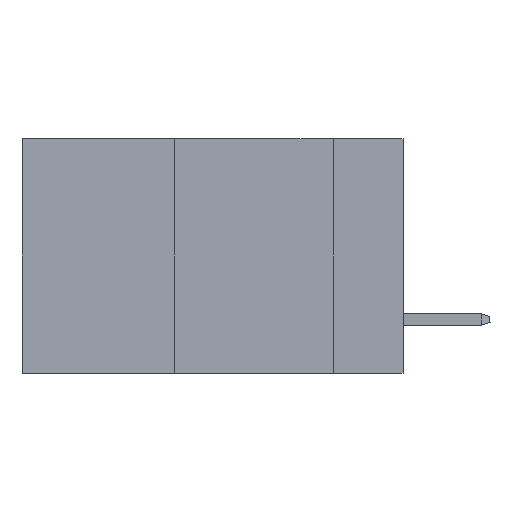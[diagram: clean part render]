
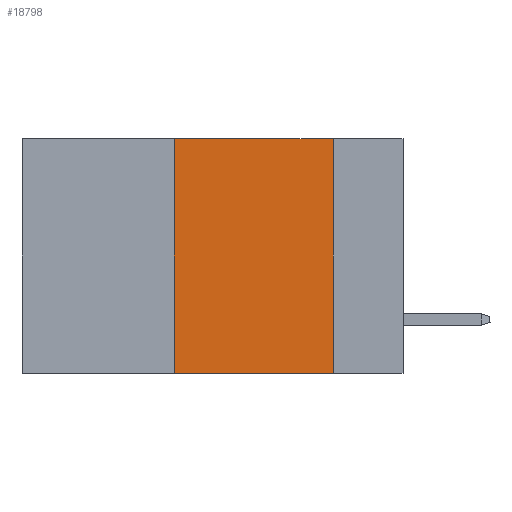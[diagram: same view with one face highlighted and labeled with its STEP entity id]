
A CAD part, left-side view. The second image highlights one B-rep face of the part: STEP entity #18798.
In plain terms, the highlighted planar face has unit normal (-1, 0, 0).
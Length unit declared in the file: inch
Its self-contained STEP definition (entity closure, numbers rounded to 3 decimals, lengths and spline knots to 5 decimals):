
#100 = LINE ( 'NONE', #15727, #6165 ) ;
#3277 = DIRECTION ( 'NONE',  ( 0., -1., 0. ) ) ;
#4380 = PLANE ( 'NONE',  #4924 ) ;
#4924 = AXIS2_PLACEMENT_3D ( 'NONE', #28492, #10896, #6681 ) ;
#5595 = VERTEX_POINT ( 'NONE', #6191 ) ;
#5866 = LINE ( 'NONE', #19051, #7879 ) ;
#6165 = VECTOR ( 'NONE', #15578, 39.37008 ) ;
#6191 = CARTESIAN_POINT ( 'NONE',  ( 0., 0.36, -0.37 ) ) ;
#6681 = DIRECTION ( 'NONE',  ( 0., 0., -1. ) ) ;
#7879 = VECTOR ( 'NONE', #21100, 39.37008 ) ;
#7904 = CARTESIAN_POINT ( 'NONE',  ( 0., 0.11, -0.37 ) ) ;
#8152 = VECTOR ( 'NONE', #3277, 39.37008 ) ;
#10287 = VERTEX_POINT ( 'NONE', #7904 ) ;
#10839 = VERTEX_POINT ( 'NONE', #17663 ) ;
#10896 = DIRECTION ( 'NONE',  ( 1., 0., 0. ) ) ;
#12550 = EDGE_CURVE ( 'NONE', #13543, #10287, #23526, .T. ) ;
#12761 = ORIENTED_EDGE ( 'NONE', *, *, #14331, .F. ) ;
#13543 = VERTEX_POINT ( 'NONE', #17713 ) ;
#14331 = EDGE_CURVE ( 'NONE', #5595, #10839, #5866, .T. ) ;
#14941 = DIRECTION ( 'NONE',  ( 0., 0., -1. ) ) ;
#15578 = DIRECTION ( 'NONE',  ( 0., -1., 0. ) ) ;
#15727 = CARTESIAN_POINT ( 'NONE',  ( 0., 0.6, -0.37 ) ) ;
#16465 = VECTOR ( 'NONE', #14941, 39.37008 ) ;
#17054 = EDGE_LOOP ( 'NONE', ( #23819, #21309, #12761, #20514 ) ) ;
#17300 = EDGE_CURVE ( 'NONE', #10839, #13543, #27406, .T. ) ;
#17663 = CARTESIAN_POINT ( 'NONE',  ( 0., 0.36, 0. ) ) ;
#17713 = CARTESIAN_POINT ( 'NONE',  ( 0., 0.11, 0. ) ) ;
#18798 = ADVANCED_FACE ( 'NONE', ( #20019 ), #4380, .F. ) ;
#19051 = CARTESIAN_POINT ( 'NONE',  ( 0., 0.36, 0. ) ) ;
#20019 = FACE_OUTER_BOUND ( 'NONE', #17054, .T. ) ;
#20514 = ORIENTED_EDGE ( 'NONE', *, *, #27109, .T. ) ;
#21100 = DIRECTION ( 'NONE',  ( 0., 0., 1. ) ) ;
#21309 = ORIENTED_EDGE ( 'NONE', *, *, #17300, .F. ) ;
#21471 = CARTESIAN_POINT ( 'NONE',  ( 0., 0.11, 0. ) ) ;
#23526 = LINE ( 'NONE', #21471, #16465 ) ;
#23819 = ORIENTED_EDGE ( 'NONE', *, *, #12550, .F. ) ;
#27109 = EDGE_CURVE ( 'NONE', #5595, #10287, #100, .T. ) ;
#27406 = LINE ( 'NONE', #27840, #8152 ) ;
#27840 = CARTESIAN_POINT ( 'NONE',  ( 0., 0.6, 0. ) ) ;
#28492 = CARTESIAN_POINT ( 'NONE',  ( 0., 0.6, 0. ) ) ;
